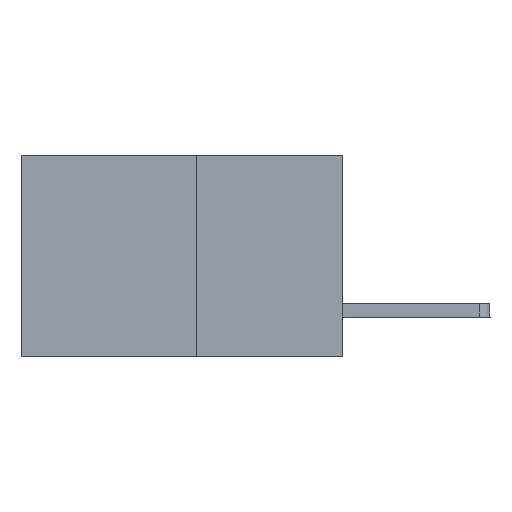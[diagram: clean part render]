
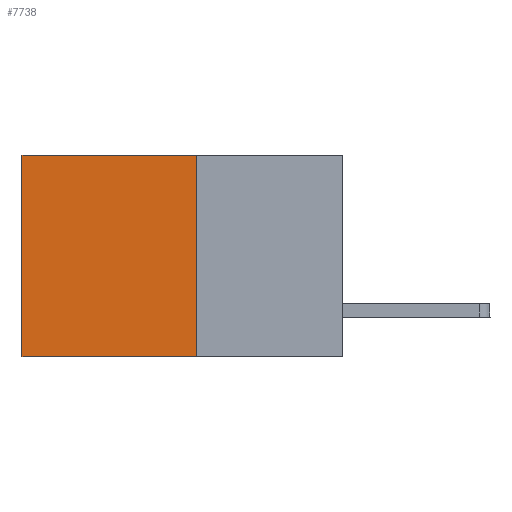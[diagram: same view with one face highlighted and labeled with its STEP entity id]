
A CAD part, left-side view. The second image highlights one B-rep face of the part: STEP entity #7738.
In plain terms, the highlighted planar face has unit normal (-1, 0, 0).
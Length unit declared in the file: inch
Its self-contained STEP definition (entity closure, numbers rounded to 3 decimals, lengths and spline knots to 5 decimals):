
#1071 = DIRECTION ( 'NONE',  ( 0., 1., 0. ) ) ;
#1283 = LINE ( 'NONE', #4907, #8433 ) ;
#2146 = VERTEX_POINT ( 'NONE', #2191 ) ;
#2191 = CARTESIAN_POINT ( 'NONE',  ( 0.277, 0.59, 0. ) ) ;
#2554 = AXIS2_PLACEMENT_3D ( 'NONE', #4188, #10467, #7807 ) ;
#2696 = ORIENTED_EDGE ( 'NONE', *, *, #6841, .F. ) ;
#2804 = ORIENTED_EDGE ( 'NONE', *, *, #3582, .T. ) ;
#2997 = VERTEX_POINT ( 'NONE', #5949 ) ;
#3117 = CARTESIAN_POINT ( 'NONE',  ( 0.277, 0.27, 0. ) ) ;
#3272 = ORIENTED_EDGE ( 'NONE', *, *, #11481, .T. ) ;
#3582 = EDGE_CURVE ( 'NONE', #2146, #2997, #8798, .T. ) ;
#4187 = ORIENTED_EDGE ( 'NONE', *, *, #7157, .F. ) ;
#4188 = CARTESIAN_POINT ( 'NONE',  ( 0.277, 0.27, -0.37 ) ) ;
#4264 = LINE ( 'NONE', #11499, #11290 ) ;
#4564 = CARTESIAN_POINT ( 'NONE',  ( 0.277, 0.27, -0.37 ) ) ;
#4907 = CARTESIAN_POINT ( 'NONE',  ( 0.277, 0.27, -0.37 ) ) ;
#5106 = DIRECTION ( 'NONE',  ( 0., 1., 0. ) ) ;
#5224 = DIRECTION ( 'NONE',  ( 0., 0., -1. ) ) ;
#5473 = CARTESIAN_POINT ( 'NONE',  ( 0.277, 0.27, 0. ) ) ;
#5949 = CARTESIAN_POINT ( 'NONE',  ( 0.277, 0.59, -0.37 ) ) ;
#6281 = CARTESIAN_POINT ( 'NONE',  ( 0.277, 0.59, -0.37 ) ) ;
#6841 = EDGE_CURVE ( 'NONE', #8232, #2997, #4264, .T. ) ;
#6851 = PLANE ( 'NONE',  #2554 ) ;
#7157 = EDGE_CURVE ( 'NONE', #8973, #8232, #1283, .T. ) ;
#7738 = ADVANCED_FACE ( 'NONE', ( #10742 ), #6851, .F. ) ;
#7807 = DIRECTION ( 'NONE',  ( 0., 0., -1. ) ) ;
#8125 = VECTOR ( 'NONE', #5224, 39.37008 ) ;
#8232 = VERTEX_POINT ( 'NONE', #4564 ) ;
#8433 = VECTOR ( 'NONE', #11240, 39.37008 ) ;
#8798 = LINE ( 'NONE', #6281, #8125 ) ;
#8973 = VERTEX_POINT ( 'NONE', #3117 ) ;
#10467 = DIRECTION ( 'NONE',  ( 1., 0., 0. ) ) ;
#10741 = VECTOR ( 'NONE', #1071, 39.37008 ) ;
#10742 = FACE_OUTER_BOUND ( 'NONE', #11396, .T. ) ;
#11084 = LINE ( 'NONE', #5473, #10741 ) ;
#11240 = DIRECTION ( 'NONE',  ( 0., 0., -1. ) ) ;
#11290 = VECTOR ( 'NONE', #5106, 39.37008 ) ;
#11396 = EDGE_LOOP ( 'NONE', ( #2804, #2696, #4187, #3272 ) ) ;
#11481 = EDGE_CURVE ( 'NONE', #8973, #2146, #11084, .T. ) ;
#11499 = CARTESIAN_POINT ( 'NONE',  ( 0.277, 0.27, -0.37 ) ) ;
